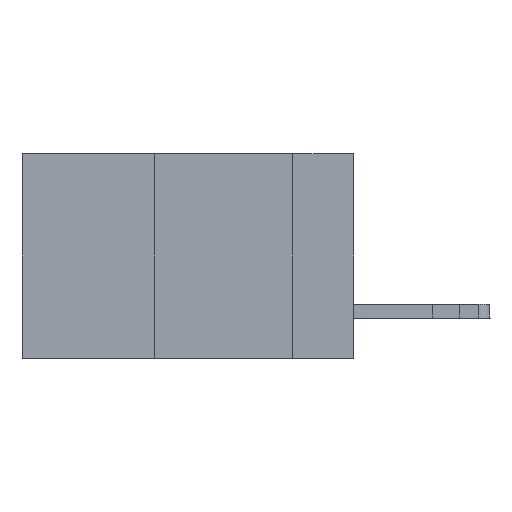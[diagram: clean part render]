
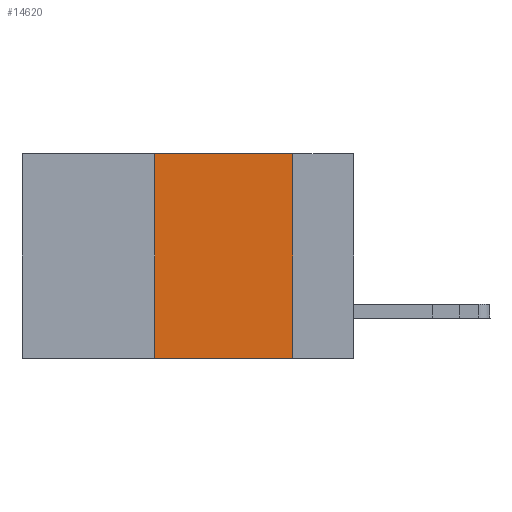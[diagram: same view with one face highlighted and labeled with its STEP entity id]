
A CAD part, left-side view. The second image highlights one B-rep face of the part: STEP entity #14620.
In plain terms, the highlighted planar face has unit normal (-1, 0, 0).
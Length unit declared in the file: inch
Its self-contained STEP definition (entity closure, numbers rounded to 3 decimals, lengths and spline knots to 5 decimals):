
#713 = CARTESIAN_POINT ( 'NONE',  ( 0., 0.6, -0.37 ) ) ;
#766 = VERTEX_POINT ( 'NONE', #3388 ) ;
#1107 = CARTESIAN_POINT ( 'NONE',  ( 0., 0.36, -0.37 ) ) ;
#2153 = LINE ( 'NONE', #19032, #13664 ) ;
#3388 = CARTESIAN_POINT ( 'NONE',  ( 0., 0.11, 0. ) ) ;
#6018 = PLANE ( 'NONE',  #19381 ) ;
#7036 = VECTOR ( 'NONE', #7418, 39.37008 ) ;
#7418 = DIRECTION ( 'NONE',  ( 0., 0., -1. ) ) ;
#8359 = CARTESIAN_POINT ( 'NONE',  ( 0., 0.6, 0. ) ) ;
#8848 = DIRECTION ( 'NONE',  ( 0., 0., 1. ) ) ;
#9206 = FACE_OUTER_BOUND ( 'NONE', #21761, .T. ) ;
#9648 = DIRECTION ( 'NONE',  ( 1., 0., 0. ) ) ;
#10078 = CARTESIAN_POINT ( 'NONE',  ( 0., 0.11, -0.37 ) ) ;
#10359 = VERTEX_POINT ( 'NONE', #10078 ) ;
#11023 = EDGE_CURVE ( 'NONE', #766, #10359, #21345, .T. ) ;
#11249 = ORIENTED_EDGE ( 'NONE', *, *, #17703, .T. ) ;
#11524 = DIRECTION ( 'NONE',  ( 0., -1., 0. ) ) ;
#11909 = VECTOR ( 'NONE', #14537, 39.37008 ) ;
#13664 = VECTOR ( 'NONE', #8848, 39.37008 ) ;
#14051 = ORIENTED_EDGE ( 'NONE', *, *, #11023, .F. ) ;
#14537 = DIRECTION ( 'NONE',  ( 0., -1., 0. ) ) ;
#14620 = ADVANCED_FACE ( 'NONE', ( #9206 ), #6018, .F. ) ;
#14749 = ORIENTED_EDGE ( 'NONE', *, *, #17537, .F. ) ;
#14763 = CARTESIAN_POINT ( 'NONE',  ( 0., 0.11, 0. ) ) ;
#15497 = VECTOR ( 'NONE', #11524, 39.37008 ) ;
#16200 = EDGE_CURVE ( 'NONE', #18710, #21358, #2153, .T. ) ;
#16223 = LINE ( 'NONE', #713, #11909 ) ;
#16537 = CARTESIAN_POINT ( 'NONE',  ( 0., 0.6, 0. ) ) ;
#16879 = ORIENTED_EDGE ( 'NONE', *, *, #16200, .F. ) ;
#16952 = LINE ( 'NONE', #8359, #15497 ) ;
#17537 = EDGE_CURVE ( 'NONE', #21358, #766, #16952, .T. ) ;
#17703 = EDGE_CURVE ( 'NONE', #18710, #10359, #16223, .T. ) ;
#18710 = VERTEX_POINT ( 'NONE', #1107 ) ;
#19032 = CARTESIAN_POINT ( 'NONE',  ( 0., 0.36, 0. ) ) ;
#19381 = AXIS2_PLACEMENT_3D ( 'NONE', #16537, #9648, #21310 ) ;
#20759 = CARTESIAN_POINT ( 'NONE',  ( 0., 0.36, 0. ) ) ;
#21310 = DIRECTION ( 'NONE',  ( 0., 0., -1. ) ) ;
#21345 = LINE ( 'NONE', #14763, #7036 ) ;
#21358 = VERTEX_POINT ( 'NONE', #20759 ) ;
#21761 = EDGE_LOOP ( 'NONE', ( #14051, #14749, #16879, #11249 ) ) ;
